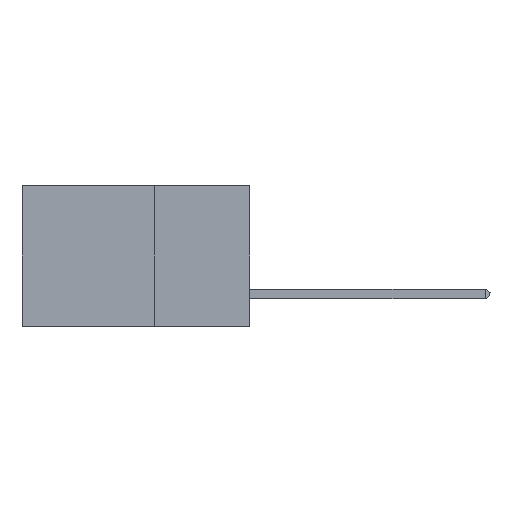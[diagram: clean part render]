
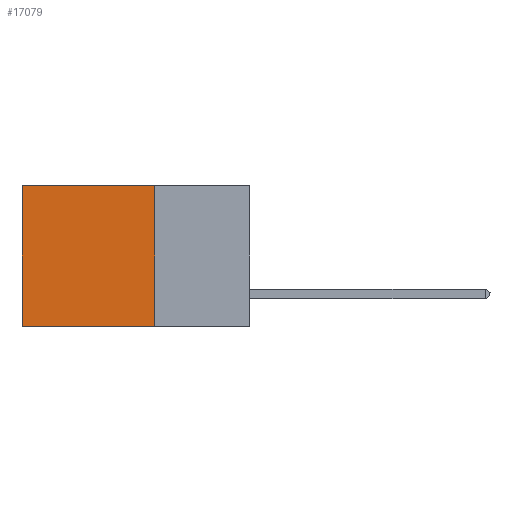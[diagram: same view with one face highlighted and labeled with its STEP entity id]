
A CAD part, left-side view. The second image highlights one B-rep face of the part: STEP entity #17079.
In plain terms, the highlighted planar face has unit normal (-1, 0, 0).
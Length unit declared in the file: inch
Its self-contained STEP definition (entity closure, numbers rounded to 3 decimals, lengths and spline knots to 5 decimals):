
#2677 = DIRECTION ( 'NONE',  ( 0., 0., -1. ) ) ;
#2709 = DIRECTION ( 'NONE',  ( 0., 1., 0. ) ) ;
#3551 = DIRECTION ( 'NONE',  ( 0., 0., -1. ) ) ;
#3675 = CARTESIAN_POINT ( 'NONE',  ( 0.2875, 0.25, 0. ) ) ;
#3864 = CARTESIAN_POINT ( 'NONE',  ( 0.2875, 0.25, 0. ) ) ;
#6180 = CARTESIAN_POINT ( 'NONE',  ( 0.2875, 0.6, -0.37 ) ) ;
#6364 = CARTESIAN_POINT ( 'NONE',  ( 0.2875, 0.25, -0.37 ) ) ;
#8683 = EDGE_CURVE ( 'NONE', #33189, #17644, #26498, .T. ) ;
#8984 = ORIENTED_EDGE ( 'NONE', *, *, #15341, .F. ) ;
#11894 = ORIENTED_EDGE ( 'NONE', *, *, #33978, .T. ) ;
#12203 = LINE ( 'NONE', #20102, #13297 ) ;
#12537 = EDGE_CURVE ( 'NONE', #41815, #21008, #24023, .T. ) ;
#12813 = CARTESIAN_POINT ( 'NONE',  ( 0.2875, 0.25, 0. ) ) ;
#13297 = VECTOR ( 'NONE', #45015, 39.37008 ) ;
#15341 = EDGE_CURVE ( 'NONE', #21008, #17644, #12203, .T. ) ;
#17079 = ADVANCED_FACE ( 'NONE', ( #41379 ), #42722, .F. ) ;
#17110 = VECTOR ( 'NONE', #2709, 39.37008 ) ;
#17644 = VERTEX_POINT ( 'NONE', #6180 ) ;
#19256 = EDGE_LOOP ( 'NONE', ( #35035, #8984, #24207, #11894 ) ) ;
#20102 = CARTESIAN_POINT ( 'NONE',  ( 0.2875, 0.25, -0.37 ) ) ;
#20154 = CARTESIAN_POINT ( 'NONE',  ( 0.2875, 0.25, 0. ) ) ;
#20940 = VECTOR ( 'NONE', #22342, 39.37008 ) ;
#21008 = VERTEX_POINT ( 'NONE', #6364 ) ;
#22342 = DIRECTION ( 'NONE',  ( 0., 0., -1. ) ) ;
#24023 = LINE ( 'NONE', #20154, #39530 ) ;
#24207 = ORIENTED_EDGE ( 'NONE', *, *, #12537, .F. ) ;
#24746 = DIRECTION ( 'NONE',  ( 1., 0., 0. ) ) ;
#25154 = CARTESIAN_POINT ( 'NONE',  ( 0.2875, 0.6, 0. ) ) ;
#26498 = LINE ( 'NONE', #25154, #20940 ) ;
#26742 = CARTESIAN_POINT ( 'NONE',  ( 0.2875, 0.6, 0. ) ) ;
#29291 = LINE ( 'NONE', #12813, #17110 ) ;
#33189 = VERTEX_POINT ( 'NONE', #26742 ) ;
#33978 = EDGE_CURVE ( 'NONE', #41815, #33189, #29291, .T. ) ;
#35035 = ORIENTED_EDGE ( 'NONE', *, *, #8683, .T. ) ;
#39530 = VECTOR ( 'NONE', #2677, 39.37008 ) ;
#39709 = AXIS2_PLACEMENT_3D ( 'NONE', #3864, #24746, #3551 ) ;
#41379 = FACE_OUTER_BOUND ( 'NONE', #19256, .T. ) ;
#41815 = VERTEX_POINT ( 'NONE', #3675 ) ;
#42722 = PLANE ( 'NONE',  #39709 ) ;
#45015 = DIRECTION ( 'NONE',  ( 0., 1., 0. ) ) ;
